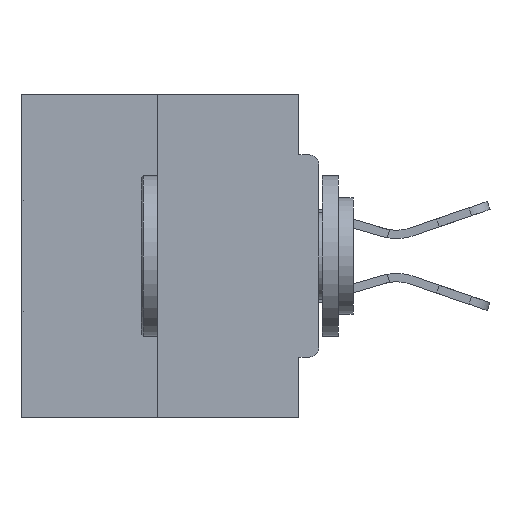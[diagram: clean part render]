
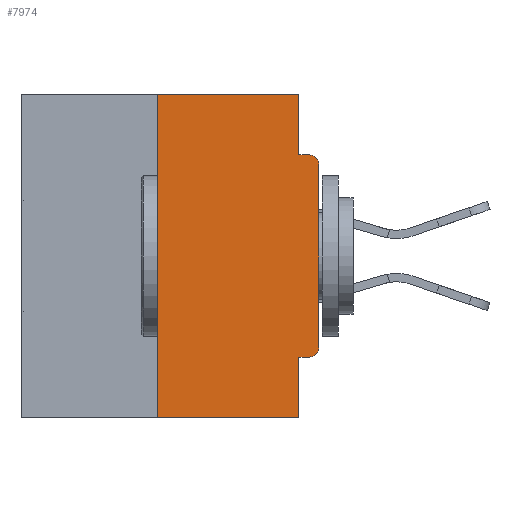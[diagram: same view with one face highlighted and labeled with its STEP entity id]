
A CAD part, left-side view. The second image highlights one B-rep face of the part: STEP entity #7974.
In plain terms, the highlighted planar face has unit normal (-1, 0, 0).
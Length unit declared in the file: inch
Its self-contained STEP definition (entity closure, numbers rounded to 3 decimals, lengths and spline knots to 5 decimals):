
#303 = CARTESIAN_POINT ( 'NONE',  ( 0., 0.25, 0. ) ) ;
#479 = LINE ( 'NONE', #38878, #24851 ) ;
#982 = CARTESIAN_POINT ( 'NONE',  ( 0., 0., -0.0935 ) ) ;
#1251 = VERTEX_POINT ( 'NONE', #40072 ) ;
#1554 = FACE_OUTER_BOUND ( 'NONE', #39903, .T. ) ;
#1934 = VECTOR ( 'NONE', #14908, 39.37008 ) ;
#1972 = EDGE_CURVE ( 'NONE', #10993, #34507, #14151, .T. ) ;
#2188 = CARTESIAN_POINT ( 'NONE',  ( 0., 0.25, 0. ) ) ;
#2211 = CARTESIAN_POINT ( 'NONE',  ( 0., 0.031, -0.0935 ) ) ;
#2387 = LINE ( 'NONE', #33255, #24766 ) ;
#2700 = AXIS2_PLACEMENT_3D ( 'NONE', #30309, #36785, #39725 ) ;
#3905 = DIRECTION ( 'NONE',  ( 0., 0., -1. ) ) ;
#4883 = VERTEX_POINT ( 'NONE', #22967 ) ;
#6520 = VECTOR ( 'NONE', #12061, 39.37008 ) ;
#6676 = LINE ( 'NONE', #22392, #22525 ) ;
#6886 = DIRECTION ( 'NONE',  ( 0., 0., -1. ) ) ;
#7974 = ADVANCED_FACE ( 'NONE', ( #1554 ), #16315, .F. ) ;
#8194 = ORIENTED_EDGE ( 'NONE', *, *, #26904, .F. ) ;
#8359 = ORIENTED_EDGE ( 'NONE', *, *, #35896, .F. ) ;
#8871 = CARTESIAN_POINT ( 'NONE',  ( 0., 0.46, -0.5 ) ) ;
#9479 = AXIS2_PLACEMENT_3D ( 'NONE', #35633, #26077, #29296 ) ;
#9660 = VECTOR ( 'NONE', #32888, 39.37008 ) ;
#10954 = ORIENTED_EDGE ( 'NONE', *, *, #39723, .F. ) ;
#10993 = VERTEX_POINT ( 'NONE', #32338 ) ;
#11103 = EDGE_CURVE ( 'NONE', #24560, #18220, #21201, .T. ) ;
#11135 = DIRECTION ( 'NONE',  ( 0., 1., 0. ) ) ;
#11212 = EDGE_CURVE ( 'NONE', #1251, #14172, #20222, .T. ) ;
#12061 = DIRECTION ( 'NONE',  ( 0., -1., 0. ) ) ;
#12477 = ORIENTED_EDGE ( 'NONE', *, *, #19016, .T. ) ;
#12855 = CARTESIAN_POINT ( 'NONE',  ( 0., 0.031, -0.5 ) ) ;
#13803 = ORIENTED_EDGE ( 'NONE', *, *, #14951, .T. ) ;
#14151 = LINE ( 'NONE', #303, #28100 ) ;
#14172 = VERTEX_POINT ( 'NONE', #18960 ) ;
#14684 = EDGE_CURVE ( 'NONE', #10993, #21542, #33966, .T. ) ;
#14908 = DIRECTION ( 'NONE',  ( 0., 0., 1. ) ) ;
#14951 = EDGE_CURVE ( 'NONE', #1251, #19879, #17954, .T. ) ;
#15870 = DIRECTION ( 'NONE',  ( 0., 0., 1. ) ) ;
#16072 = LINE ( 'NONE', #982, #9660 ) ;
#16139 = DIRECTION ( 'NONE',  ( 0., 0., -1. ) ) ;
#16315 = PLANE ( 'NONE',  #9479 ) ;
#16795 = ORIENTED_EDGE ( 'NONE', *, *, #14684, .T. ) ;
#17265 = DIRECTION ( 'NONE',  ( -1., 0., 0. ) ) ;
#17954 = CIRCLE ( 'NONE', #2700, 0.015 ) ;
#18220 = VERTEX_POINT ( 'NONE', #24736 ) ;
#18225 = VECTOR ( 'NONE', #11135, 39.37008 ) ;
#18960 = CARTESIAN_POINT ( 'NONE',  ( 0., 0.031, -0.4065 ) ) ;
#19016 = EDGE_CURVE ( 'NONE', #19879, #24560, #33339, .T. ) ;
#19589 = VERTEX_POINT ( 'NONE', #2211 ) ;
#19879 = VERTEX_POINT ( 'NONE', #37180 ) ;
#20222 = LINE ( 'NONE', #36571, #18225 ) ;
#21201 = CIRCLE ( 'NONE', #33853, 0.015 ) ;
#21542 = VERTEX_POINT ( 'NONE', #12855 ) ;
#22392 = CARTESIAN_POINT ( 'NONE',  ( 0., 0.031, -0.5 ) ) ;
#22525 = VECTOR ( 'NONE', #16139, 39.37008 ) ;
#22967 = CARTESIAN_POINT ( 'NONE',  ( 0., 0.031, 0. ) ) ;
#24560 = VERTEX_POINT ( 'NONE', #37865 ) ;
#24736 = CARTESIAN_POINT ( 'NONE',  ( 0., 0.015, -0.0935 ) ) ;
#24766 = VECTOR ( 'NONE', #27090, 39.37008 ) ;
#24851 = VECTOR ( 'NONE', #6886, 39.37008 ) ;
#25229 = ORIENTED_EDGE ( 'NONE', *, *, #39884, .F. ) ;
#25673 = ORIENTED_EDGE ( 'NONE', *, *, #1972, .F. ) ;
#26077 = DIRECTION ( 'NONE',  ( 1., 0., 0. ) ) ;
#26175 = ORIENTED_EDGE ( 'NONE', *, *, #11103, .T. ) ;
#26904 = EDGE_CURVE ( 'NONE', #34507, #4883, #2387, .T. ) ;
#27090 = DIRECTION ( 'NONE',  ( 0., -1., 0. ) ) ;
#28100 = VECTOR ( 'NONE', #15870, 39.37008 ) ;
#29214 = ORIENTED_EDGE ( 'NONE', *, *, #11212, .F. ) ;
#29296 = DIRECTION ( 'NONE',  ( 0., 0., -1. ) ) ;
#30309 = CARTESIAN_POINT ( 'NONE',  ( 0., 0.015, -0.3915 ) ) ;
#32338 = CARTESIAN_POINT ( 'NONE',  ( 0., 0.25, -0.5 ) ) ;
#32888 = DIRECTION ( 'NONE',  ( 0., -1., 0. ) ) ;
#33255 = CARTESIAN_POINT ( 'NONE',  ( 0., 0.46, 0. ) ) ;
#33339 = LINE ( 'NONE', #34467, #1934 ) ;
#33853 = AXIS2_PLACEMENT_3D ( 'NONE', #36438, #17265, #3905 ) ;
#33966 = LINE ( 'NONE', #8871, #6520 ) ;
#34467 = CARTESIAN_POINT ( 'NONE',  ( 0., 0., 0. ) ) ;
#34507 = VERTEX_POINT ( 'NONE', #2188 ) ;
#35633 = CARTESIAN_POINT ( 'NONE',  ( 0., 0.46, 0. ) ) ;
#35896 = EDGE_CURVE ( 'NONE', #4883, #19589, #479, .T. ) ;
#36438 = CARTESIAN_POINT ( 'NONE',  ( 0., 0.015, -0.1085 ) ) ;
#36571 = CARTESIAN_POINT ( 'NONE',  ( 0., 0., -0.4065 ) ) ;
#36785 = DIRECTION ( 'NONE',  ( -1., 0., 0. ) ) ;
#37180 = CARTESIAN_POINT ( 'NONE',  ( 0., 0., -0.3915 ) ) ;
#37865 = CARTESIAN_POINT ( 'NONE',  ( 0., 0., -0.1085 ) ) ;
#38878 = CARTESIAN_POINT ( 'NONE',  ( 0., 0.031, 0. ) ) ;
#39723 = EDGE_CURVE ( 'NONE', #14172, #21542, #6676, .T. ) ;
#39725 = DIRECTION ( 'NONE',  ( 0., 0., -1. ) ) ;
#39884 = EDGE_CURVE ( 'NONE', #19589, #18220, #16072, .T. ) ;
#39903 = EDGE_LOOP ( 'NONE', ( #8194, #25673, #16795, #10954, #29214, #13803, #12477, #26175, #25229, #8359 ) ) ;
#40072 = CARTESIAN_POINT ( 'NONE',  ( 0., 0.015, -0.4065 ) ) ;
